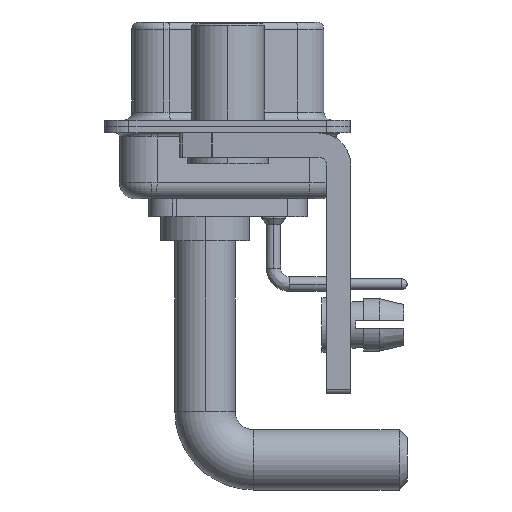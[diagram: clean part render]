
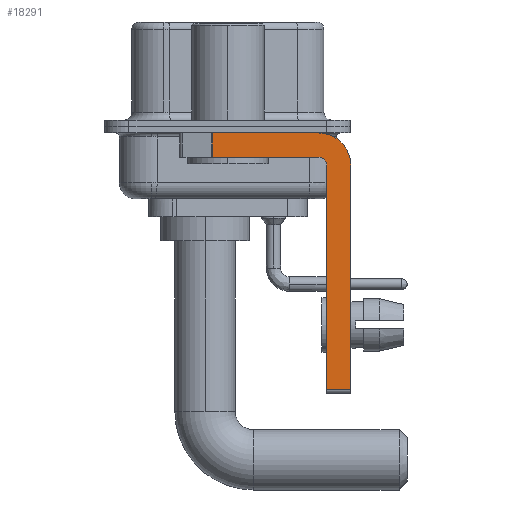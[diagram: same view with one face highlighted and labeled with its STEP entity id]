
A CAD part, left-side view. The second image highlights one B-rep face of the part: STEP entity #18291.
In plain terms, the highlighted planar face has unit normal (-1, 0, 0).
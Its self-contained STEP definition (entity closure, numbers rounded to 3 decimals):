
#127 = DIRECTION ( 'NONE',  ( 0., 0., -1. ) ) ;
#349 = VERTEX_POINT ( 'NONE', #15164 ) ;
#743 = LINE ( 'NONE', #13237, #8818 ) ;
#910 = VERTEX_POINT ( 'NONE', #20606 ) ;
#1688 = AXIS2_PLACEMENT_3D ( 'NONE', #2559, #2424, #21157 ) ;
#2246 = DIRECTION ( 'NONE',  ( 0., 0., -1. ) ) ;
#2424 = DIRECTION ( 'NONE',  ( -1., 0., 0. ) ) ;
#2515 = ORIENTED_EDGE ( 'NONE', *, *, #5443, .F. ) ;
#2559 = CARTESIAN_POINT ( 'NONE',  ( -2.9, -5.65, -2.4 ) ) ;
#2789 = CARTESIAN_POINT ( 'NONE',  ( -2.9, 0.978, -1.9 ) ) ;
#2928 = LINE ( 'NONE', #19842, #25487 ) ;
#3068 = DIRECTION ( 'NONE',  ( 0., 1., 0. ) ) ;
#3961 = LINE ( 'NONE', #14508, #8925 ) ;
#4772 = CIRCLE ( 'NONE', #1688, 0.5 ) ;
#4812 = AXIS2_PLACEMENT_3D ( 'NONE', #14761, #8232, #25458 ) ;
#5277 = VERTEX_POINT ( 'NONE', #21754 ) ;
#5443 = EDGE_CURVE ( 'NONE', #910, #22531, #3961, .T. ) ;
#7451 = VERTEX_POINT ( 'NONE', #17528 ) ;
#7467 = VERTEX_POINT ( 'NONE', #13781 ) ;
#8232 = DIRECTION ( 'NONE',  ( 1., 0., 0. ) ) ;
#8729 = CARTESIAN_POINT ( 'NONE',  ( -2.9, -6.15, -16.35 ) ) ;
#8818 = VECTOR ( 'NONE', #13516, 1000. ) ;
#8925 = VECTOR ( 'NONE', #26857, 1000. ) ;
#9053 = EDGE_CURVE ( 'NONE', #25192, #7467, #14725, .T. ) ;
#9243 = VERTEX_POINT ( 'NONE', #14865 ) ;
#9311 = EDGE_CURVE ( 'NONE', #910, #7451, #10718, .T. ) ;
#10417 = EDGE_CURVE ( 'NONE', #9243, #7451, #2928, .T. ) ;
#10430 = CARTESIAN_POINT ( 'NONE',  ( -2.9, -5.65, -16.35 ) ) ;
#10650 = ORIENTED_EDGE ( 'NONE', *, *, #26454, .F. ) ;
#10718 = LINE ( 'NONE', #2789, #17588 ) ;
#11103 = FACE_OUTER_BOUND ( 'NONE', #19348, .T. ) ;
#11238 = DIRECTION ( 'NONE',  ( 1., 0., 0. ) ) ;
#11476 = CIRCLE ( 'NONE', #4812, 2. ) ;
#12603 = LINE ( 'NONE', #16756, #22983 ) ;
#13237 = CARTESIAN_POINT ( 'NONE',  ( -2.9, -6.15, -16.6 ) ) ;
#13516 = DIRECTION ( 'NONE',  ( 0., 0., 1. ) ) ;
#13781 = CARTESIAN_POINT ( 'NONE',  ( -2.9, -7.65, -16.35 ) ) ;
#13943 = CARTESIAN_POINT ( 'NONE',  ( -2.9, -5.65, -0.4 ) ) ;
#14508 = CARTESIAN_POINT ( 'NONE',  ( -2.9, 3., -0.4 ) ) ;
#14608 = AXIS2_PLACEMENT_3D ( 'NONE', #23728, #11238, #15138 ) ;
#14725 = LINE ( 'NONE', #10430, #16994 ) ;
#14761 = CARTESIAN_POINT ( 'NONE',  ( -2.9, -5.65, -2.4 ) ) ;
#14865 = CARTESIAN_POINT ( 'NONE',  ( -2.9, -5.65, -1.9 ) ) ;
#15138 = DIRECTION ( 'NONE',  ( 0., 0., -1. ) ) ;
#15164 = CARTESIAN_POINT ( 'NONE',  ( -2.9, -7.65, -2.4 ) ) ;
#16756 = CARTESIAN_POINT ( 'NONE',  ( -2.9, -7.65, -2.4 ) ) ;
#16819 = DIRECTION ( 'NONE',  ( 0., -1., 0. ) ) ;
#16994 = VECTOR ( 'NONE', #16819, 1000. ) ;
#17126 = EDGE_CURVE ( 'NONE', #349, #7467, #12603, .T. ) ;
#17500 = ORIENTED_EDGE ( 'NONE', *, *, #17126, .F. ) ;
#17528 = CARTESIAN_POINT ( 'NONE',  ( -2.9, 0.978, -1.9 ) ) ;
#17588 = VECTOR ( 'NONE', #2246, 1000. ) ;
#17612 = PLANE ( 'NONE',  #14608 ) ;
#17762 = ORIENTED_EDGE ( 'NONE', *, *, #9311, .T. ) ;
#18291 = ADVANCED_FACE ( 'NONE', ( #11103 ), #17612, .F. ) ;
#19348 = EDGE_LOOP ( 'NONE', ( #2515, #17762, #24433, #21903, #20807, #20232, #17500, #10650 ) ) ;
#19842 = CARTESIAN_POINT ( 'NONE',  ( -2.9, -5.65, -1.9 ) ) ;
#20232 = ORIENTED_EDGE ( 'NONE', *, *, #9053, .T. ) ;
#20606 = CARTESIAN_POINT ( 'NONE',  ( -2.9, 0.978, -0.4 ) ) ;
#20807 = ORIENTED_EDGE ( 'NONE', *, *, #26616, .F. ) ;
#21157 = DIRECTION ( 'NONE',  ( 0., 0., 1. ) ) ;
#21754 = CARTESIAN_POINT ( 'NONE',  ( -2.9, -6.15, -2.4 ) ) ;
#21903 = ORIENTED_EDGE ( 'NONE', *, *, #25899, .F. ) ;
#22531 = VERTEX_POINT ( 'NONE', #13943 ) ;
#22983 = VECTOR ( 'NONE', #127, 1000. ) ;
#23728 = CARTESIAN_POINT ( 'NONE',  ( -2.9, -5.65, -2.4 ) ) ;
#24433 = ORIENTED_EDGE ( 'NONE', *, *, #10417, .F. ) ;
#25192 = VERTEX_POINT ( 'NONE', #8729 ) ;
#25458 = DIRECTION ( 'NONE',  ( 0., 0., -1. ) ) ;
#25487 = VECTOR ( 'NONE', #3068, 1000. ) ;
#25899 = EDGE_CURVE ( 'NONE', #5277, #9243, #4772, .T. ) ;
#26454 = EDGE_CURVE ( 'NONE', #22531, #349, #11476, .T. ) ;
#26616 = EDGE_CURVE ( 'NONE', #25192, #5277, #743, .T. ) ;
#26857 = DIRECTION ( 'NONE',  ( 0., -1., 0. ) ) ;
